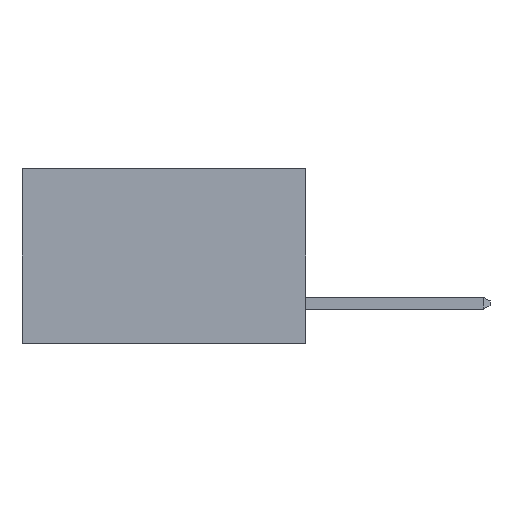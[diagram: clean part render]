
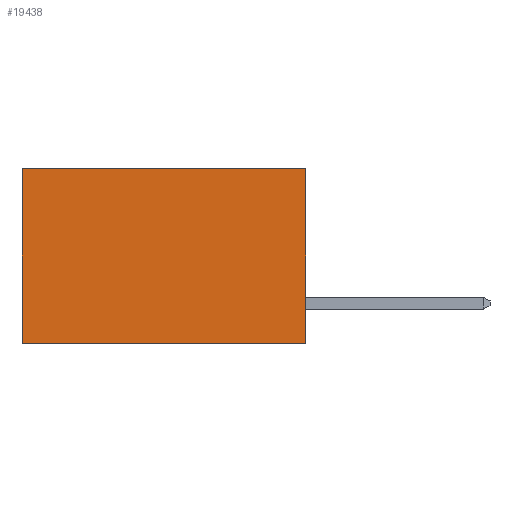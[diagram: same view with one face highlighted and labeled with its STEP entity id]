
A CAD part, left-side view. The second image highlights one B-rep face of the part: STEP entity #19438.
In plain terms, the highlighted planar face has unit normal (-1, 0, 0).
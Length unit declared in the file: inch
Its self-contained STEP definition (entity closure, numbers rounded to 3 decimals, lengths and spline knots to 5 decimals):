
#551 = ORIENTED_EDGE ( 'NONE', *, *, #3372, .F. ) ;
#568 = CARTESIAN_POINT ( 'NONE',  ( 0.298, 0., -0.37 ) ) ;
#927 = CARTESIAN_POINT ( 'NONE',  ( 0.298, 0., 0. ) ) ;
#1057 = CARTESIAN_POINT ( 'NONE',  ( 0.298, 0., 0. ) ) ;
#1480 = DIRECTION ( 'NONE',  ( 0., 0., -1. ) ) ;
#3372 = EDGE_CURVE ( 'NONE', #9122, #19151, #16891, .T. ) ;
#3550 = CARTESIAN_POINT ( 'NONE',  ( 0.298, 0.6, 0. ) ) ;
#4534 = CARTESIAN_POINT ( 'NONE',  ( 0.298, 0., 0. ) ) ;
#4577 = EDGE_CURVE ( 'NONE', #8735, #5348, #6768, .T. ) ;
#4603 = AXIS2_PLACEMENT_3D ( 'NONE', #927, #8011, #19482 ) ;
#5348 = VERTEX_POINT ( 'NONE', #3550 ) ;
#5558 = CARTESIAN_POINT ( 'NONE',  ( 0.298, 0.6, -0.37 ) ) ;
#5703 = EDGE_CURVE ( 'NONE', #8735, #9122, #17553, .T. ) ;
#6768 = LINE ( 'NONE', #17137, #16060 ) ;
#8011 = DIRECTION ( 'NONE',  ( 1., 0., 0. ) ) ;
#8258 = VECTOR ( 'NONE', #1480, 39.37008 ) ;
#8735 = VERTEX_POINT ( 'NONE', #1057 ) ;
#9122 = VERTEX_POINT ( 'NONE', #568 ) ;
#9250 = FACE_OUTER_BOUND ( 'NONE', #21632, .T. ) ;
#10388 = CARTESIAN_POINT ( 'NONE',  ( 0.298, 0., -0.37 ) ) ;
#10419 = DIRECTION ( 'NONE',  ( 0., 1., 0. ) ) ;
#10664 = DIRECTION ( 'NONE',  ( 0., 0., -1. ) ) ;
#10716 = ORIENTED_EDGE ( 'NONE', *, *, #13102, .T. ) ;
#11867 = CARTESIAN_POINT ( 'NONE',  ( 0.298, 0.6, 0. ) ) ;
#12636 = VECTOR ( 'NONE', #10419, 39.37008 ) ;
#12782 = VECTOR ( 'NONE', #10664, 39.37008 ) ;
#13015 = PLANE ( 'NONE',  #4603 ) ;
#13102 = EDGE_CURVE ( 'NONE', #5348, #19151, #15967, .T. ) ;
#14095 = ORIENTED_EDGE ( 'NONE', *, *, #4577, .T. ) ;
#15967 = LINE ( 'NONE', #11867, #8258 ) ;
#16060 = VECTOR ( 'NONE', #17116, 39.37008 ) ;
#16891 = LINE ( 'NONE', #10388, #12636 ) ;
#17116 = DIRECTION ( 'NONE',  ( 0., 1., 0. ) ) ;
#17137 = CARTESIAN_POINT ( 'NONE',  ( 0.298, 0., 0. ) ) ;
#17553 = LINE ( 'NONE', #4534, #12782 ) ;
#19151 = VERTEX_POINT ( 'NONE', #5558 ) ;
#19438 = ADVANCED_FACE ( 'NONE', ( #9250 ), #13015, .F. ) ;
#19482 = DIRECTION ( 'NONE',  ( 0., 0., -1. ) ) ;
#19508 = ORIENTED_EDGE ( 'NONE', *, *, #5703, .F. ) ;
#21632 = EDGE_LOOP ( 'NONE', ( #10716, #551, #19508, #14095 ) ) ;
